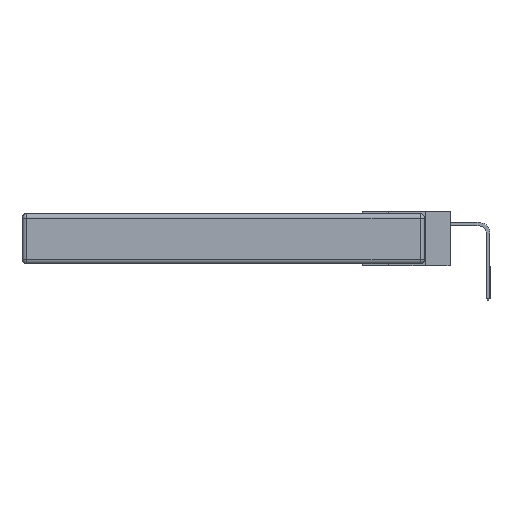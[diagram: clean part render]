
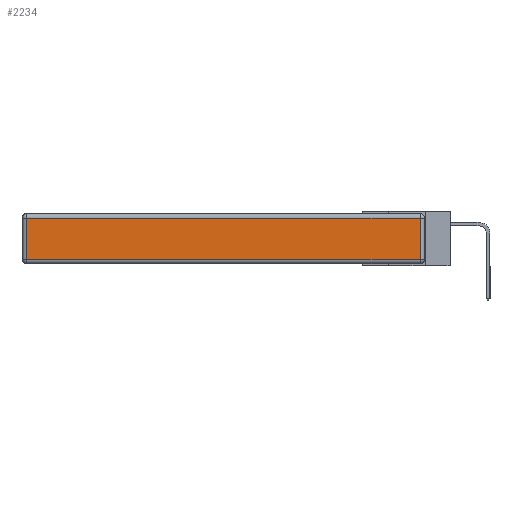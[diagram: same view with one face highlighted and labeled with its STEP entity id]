
A CAD part, left-side view. The second image highlights one B-rep face of the part: STEP entity #2234.
In plain terms, the highlighted planar face has unit normal (-1, 0, 0).
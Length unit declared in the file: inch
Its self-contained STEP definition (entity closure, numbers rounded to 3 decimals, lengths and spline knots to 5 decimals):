
#39 = PLANE ( 'NONE',  #22141 ) ;
#919 = VECTOR ( 'NONE', #1165, 39.37008 ) ;
#1165 = DIRECTION ( 'NONE',  ( 0., 0., 1. ) ) ;
#2231 = VERTEX_POINT ( 'NONE', #5645 ) ;
#2234 = ADVANCED_FACE ( 'NONE', ( #11560 ), #39, .T. ) ;
#2332 = CARTESIAN_POINT ( 'NONE',  ( 0., 2.72, -0.343 ) ) ;
#5145 = CARTESIAN_POINT ( 'NONE',  ( 0., 2.72, -0.03 ) ) ;
#5645 = CARTESIAN_POINT ( 'NONE',  ( 0., 0.03, -0.313 ) ) ;
#6368 = VERTEX_POINT ( 'NONE', #5145 ) ;
#7368 = LINE ( 'NONE', #10351, #20919 ) ;
#7474 = VECTOR ( 'NONE', #17815, 39.37008 ) ;
#7742 = DIRECTION ( 'NONE',  ( 0., 0., 1. ) ) ;
#7894 = CARTESIAN_POINT ( 'NONE',  ( 0., 0.03, -0.03 ) ) ;
#8257 = EDGE_CURVE ( 'NONE', #18479, #6368, #22523, .T. ) ;
#8319 = ORIENTED_EDGE ( 'NONE', *, *, #8257, .T. ) ;
#8742 = ORIENTED_EDGE ( 'NONE', *, *, #14805, .T. ) ;
#9377 = VECTOR ( 'NONE', #12010, 39.37008 ) ;
#9501 = VERTEX_POINT ( 'NONE', #21164 ) ;
#10351 = CARTESIAN_POINT ( 'NONE',  ( 0., 0., -0.313 ) ) ;
#10393 = ORIENTED_EDGE ( 'NONE', *, *, #22571, .T. ) ;
#11560 = FACE_OUTER_BOUND ( 'NONE', #17463, .T. ) ;
#11682 = CARTESIAN_POINT ( 'NONE',  ( 0., 0., -0.343 ) ) ;
#12000 = CARTESIAN_POINT ( 'NONE',  ( 0., 2.75, -0.03 ) ) ;
#12010 = DIRECTION ( 'NONE',  ( 0., 0., -1. ) ) ;
#12190 = DIRECTION ( 'NONE',  ( 0., -1., 0. ) ) ;
#12721 = CARTESIAN_POINT ( 'NONE',  ( 0., 0.03, -0.343 ) ) ;
#14805 = EDGE_CURVE ( 'NONE', #2231, #18479, #21463, .T. ) ;
#17463 = EDGE_LOOP ( 'NONE', ( #10393, #8742, #8319, #23288 ) ) ;
#17815 = DIRECTION ( 'NONE',  ( 0., 1., 0. ) ) ;
#18479 = VERTEX_POINT ( 'NONE', #7894 ) ;
#19119 = DIRECTION ( 'NONE',  ( -1., 0., 0. ) ) ;
#19337 = LINE ( 'NONE', #2332, #9377 ) ;
#20919 = VECTOR ( 'NONE', #12190, 39.37008 ) ;
#21164 = CARTESIAN_POINT ( 'NONE',  ( 0., 2.72, -0.313 ) ) ;
#21463 = LINE ( 'NONE', #12721, #919 ) ;
#22141 = AXIS2_PLACEMENT_3D ( 'NONE', #11682, #19119, #7742 ) ;
#22523 = LINE ( 'NONE', #12000, #7474 ) ;
#22571 = EDGE_CURVE ( 'NONE', #9501, #2231, #7368, .T. ) ;
#23288 = ORIENTED_EDGE ( 'NONE', *, *, #24669, .T. ) ;
#24669 = EDGE_CURVE ( 'NONE', #6368, #9501, #19337, .T. ) ;
